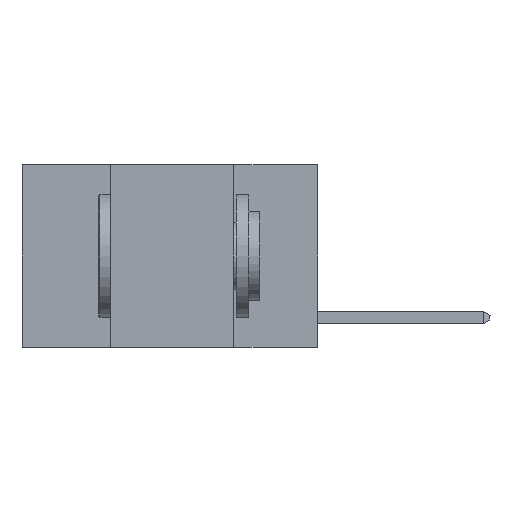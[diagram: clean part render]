
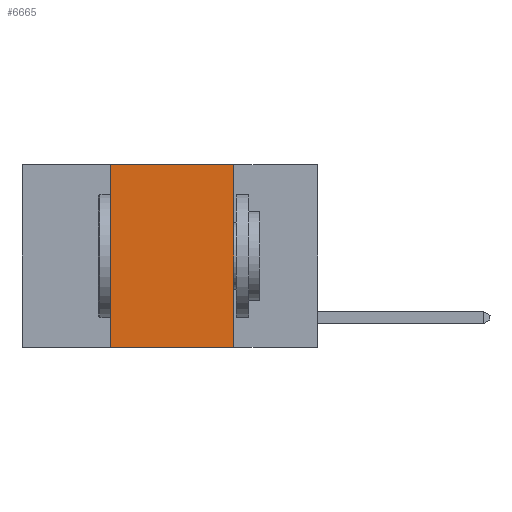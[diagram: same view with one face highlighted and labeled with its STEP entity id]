
A CAD part, left-side view. The second image highlights one B-rep face of the part: STEP entity #6665.
In plain terms, the highlighted planar face has unit normal (-1, 0, 0).
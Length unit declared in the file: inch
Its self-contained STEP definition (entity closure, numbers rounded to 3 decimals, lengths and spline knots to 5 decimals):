
#72 = LINE ( 'NONE', #11929, #6907 ) ;
#450 = DIRECTION ( 'NONE',  ( 0., -1., 0. ) ) ;
#810 = EDGE_LOOP ( 'NONE', ( #11877, #11817, #11579, #10920 ) ) ;
#1011 = AXIS2_PLACEMENT_3D ( 'NONE', #12142, #9784, #13416 ) ;
#1503 = EDGE_CURVE ( 'NONE', #2315, #4423, #11096, .T. ) ;
#2162 = EDGE_CURVE ( 'NONE', #8384, #11257, #8176, .T. ) ;
#2315 = VERTEX_POINT ( 'NONE', #8074 ) ;
#2638 = CARTESIAN_POINT ( 'NONE',  ( 0., 0.17, -0.37 ) ) ;
#4423 = VERTEX_POINT ( 'NONE', #2638 ) ;
#6665 = ADVANCED_FACE ( 'NONE', ( #13054 ), #7321, .F. ) ;
#6816 = VECTOR ( 'NONE', #11716, 39.37008 ) ;
#6907 = VECTOR ( 'NONE', #6959, 39.37008 ) ;
#6959 = DIRECTION ( 'NONE',  ( 0., -1., 0. ) ) ;
#7002 = VECTOR ( 'NONE', #8653, 39.37008 ) ;
#7019 = EDGE_CURVE ( 'NONE', #11257, #2315, #13648, .T. ) ;
#7031 = CARTESIAN_POINT ( 'NONE',  ( 0., 0.42, -0.37 ) ) ;
#7050 = CARTESIAN_POINT ( 'NONE',  ( 0., 0.6, 0. ) ) ;
#7321 = PLANE ( 'NONE',  #1011 ) ;
#7738 = CARTESIAN_POINT ( 'NONE',  ( 0., 0.17, 0. ) ) ;
#8074 = CARTESIAN_POINT ( 'NONE',  ( 0., 0.17, 0. ) ) ;
#8176 = LINE ( 'NONE', #13819, #7002 ) ;
#8384 = VERTEX_POINT ( 'NONE', #7031 ) ;
#8653 = DIRECTION ( 'NONE',  ( 0., 0., 1. ) ) ;
#8816 = EDGE_CURVE ( 'NONE', #8384, #4423, #72, .T. ) ;
#9784 = DIRECTION ( 'NONE',  ( 1., 0., 0. ) ) ;
#10920 = ORIENTED_EDGE ( 'NONE', *, *, #8816, .T. ) ;
#11096 = LINE ( 'NONE', #7738, #6816 ) ;
#11257 = VERTEX_POINT ( 'NONE', #14675 ) ;
#11579 = ORIENTED_EDGE ( 'NONE', *, *, #2162, .F. ) ;
#11716 = DIRECTION ( 'NONE',  ( 0., 0., -1. ) ) ;
#11817 = ORIENTED_EDGE ( 'NONE', *, *, #7019, .F. ) ;
#11877 = ORIENTED_EDGE ( 'NONE', *, *, #1503, .F. ) ;
#11929 = CARTESIAN_POINT ( 'NONE',  ( 0., 0.6, -0.37 ) ) ;
#12142 = CARTESIAN_POINT ( 'NONE',  ( 0., 0.6, 0. ) ) ;
#13054 = FACE_OUTER_BOUND ( 'NONE', #810, .T. ) ;
#13258 = VECTOR ( 'NONE', #450, 39.37008 ) ;
#13416 = DIRECTION ( 'NONE',  ( 0., 0., -1. ) ) ;
#13648 = LINE ( 'NONE', #7050, #13258 ) ;
#13819 = CARTESIAN_POINT ( 'NONE',  ( 0., 0.42, 0. ) ) ;
#14675 = CARTESIAN_POINT ( 'NONE',  ( 0., 0.42, 0. ) ) ;
